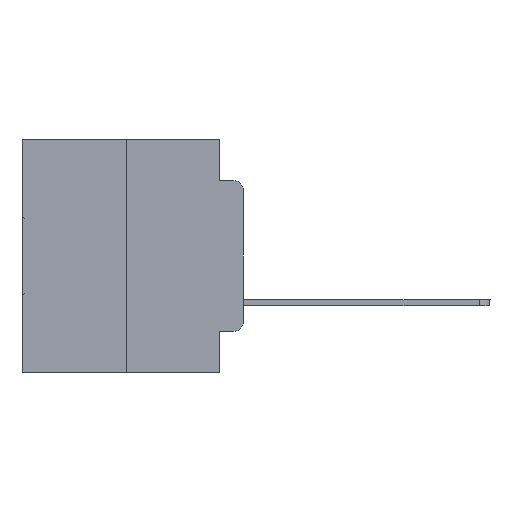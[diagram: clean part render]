
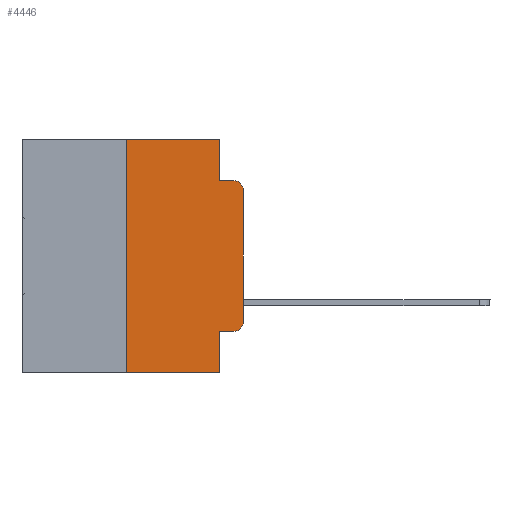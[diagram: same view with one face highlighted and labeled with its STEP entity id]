
A CAD part, left-side view. The second image highlights one B-rep face of the part: STEP entity #4446.
In plain terms, the highlighted planar face has unit normal (-1, 0, 0).
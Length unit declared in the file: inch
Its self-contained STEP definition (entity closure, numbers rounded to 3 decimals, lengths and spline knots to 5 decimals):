
#387 = VERTEX_POINT ( 'NONE', #19240 ) ;
#478 = EDGE_CURVE ( 'NONE', #12001, #10511, #5545, .T. ) ;
#784 = CARTESIAN_POINT ( 'NONE',  ( 0., 0.051, -0.4115 ) ) ;
#855 = VERTEX_POINT ( 'NONE', #19001 ) ;
#1096 = CARTESIAN_POINT ( 'NONE',  ( 0., 0.25, 0. ) ) ;
#1797 = LINE ( 'NONE', #3790, #17445 ) ;
#2346 = EDGE_CURVE ( 'NONE', #4085, #24721, #22886, .T. ) ;
#2978 = CARTESIAN_POINT ( 'NONE',  ( 0., 0.051, 0. ) ) ;
#3508 = CARTESIAN_POINT ( 'NONE',  ( 0., 0.051, 0. ) ) ;
#3790 = CARTESIAN_POINT ( 'NONE',  ( 0., 0.051, -0.0885 ) ) ;
#4085 = VERTEX_POINT ( 'NONE', #2978 ) ;
#4171 = ORIENTED_EDGE ( 'NONE', *, *, #13759, .T. ) ;
#4347 = VECTOR ( 'NONE', #24186, 39.37008 ) ;
#4446 = ADVANCED_FACE ( 'NONE', ( #16095 ), #20262, .F. ) ;
#5102 = DIRECTION ( 'NONE',  ( 0., 0., -1. ) ) ;
#5545 = LINE ( 'NONE', #1096, #15747 ) ;
#6130 = ORIENTED_EDGE ( 'NONE', *, *, #12969, .T. ) ;
#6351 = ORIENTED_EDGE ( 'NONE', *, *, #13719, .F. ) ;
#6355 = VECTOR ( 'NONE', #13452, 39.37008 ) ;
#6681 = CARTESIAN_POINT ( 'NONE',  ( 0., 0.25, -0.5 ) ) ;
#7059 = AXIS2_PLACEMENT_3D ( 'NONE', #24426, #24642, #22497 ) ;
#7614 = AXIS2_PLACEMENT_3D ( 'NONE', #11608, #21260, #5102 ) ;
#7624 = VECTOR ( 'NONE', #13855, 39.37008 ) ;
#8023 = VECTOR ( 'NONE', #24459, 39.37008 ) ;
#9468 = CARTESIAN_POINT ( 'NONE',  ( 0., 0.02, -0.1085 ) ) ;
#9555 = ORIENTED_EDGE ( 'NONE', *, *, #25316, .T. ) ;
#9809 = CARTESIAN_POINT ( 'NONE',  ( 0., 0.051, -0.4115 ) ) ;
#10511 = VERTEX_POINT ( 'NONE', #12247 ) ;
#10551 = LINE ( 'NONE', #784, #4347 ) ;
#11219 = CARTESIAN_POINT ( 'NONE',  ( 0., 0.473, -0.5 ) ) ;
#11608 = CARTESIAN_POINT ( 'NONE',  ( 0., 0.02, -0.3915 ) ) ;
#11614 = ORIENTED_EDGE ( 'NONE', *, *, #23508, .T. ) ;
#12001 = VERTEX_POINT ( 'NONE', #6681 ) ;
#12176 = DIRECTION ( 'NONE',  ( 0., 0., 1. ) ) ;
#12247 = CARTESIAN_POINT ( 'NONE',  ( 0., 0.25, 0. ) ) ;
#12268 = LINE ( 'NONE', #17048, #21388 ) ;
#12561 = VERTEX_POINT ( 'NONE', #15906 ) ;
#12969 = EDGE_CURVE ( 'NONE', #25031, #12561, #14559, .T. ) ;
#13251 = LINE ( 'NONE', #11219, #6355 ) ;
#13452 = DIRECTION ( 'NONE',  ( 0., -1., 0. ) ) ;
#13719 = EDGE_CURVE ( 'NONE', #24721, #12561, #1797, .T. ) ;
#13759 = EDGE_CURVE ( 'NONE', #27956, #27837, #10551, .T. ) ;
#13766 = VECTOR ( 'NONE', #25770, 39.37008 ) ;
#13855 = DIRECTION ( 'NONE',  ( 0., 0., -1. ) ) ;
#13918 = EDGE_LOOP ( 'NONE', ( #11614, #6130, #6351, #15587, #24100, #21765, #9555, #19678, #4171, #14757 ) ) ;
#14559 = CIRCLE ( 'NONE', #15472, 0.02 ) ;
#14757 = ORIENTED_EDGE ( 'NONE', *, *, #17914, .T. ) ;
#15472 = AXIS2_PLACEMENT_3D ( 'NONE', #9468, #25727, #21134 ) ;
#15587 = ORIENTED_EDGE ( 'NONE', *, *, #2346, .F. ) ;
#15747 = VECTOR ( 'NONE', #17697, 39.37008 ) ;
#15906 = CARTESIAN_POINT ( 'NONE',  ( 0., 0.02, -0.0885 ) ) ;
#16095 = FACE_OUTER_BOUND ( 'NONE', #13918, .T. ) ;
#16406 = CARTESIAN_POINT ( 'NONE',  ( 0., 0.02, -0.4115 ) ) ;
#16682 = LINE ( 'NONE', #25470, #13766 ) ;
#17048 = CARTESIAN_POINT ( 'NONE',  ( 0., 0., 0. ) ) ;
#17445 = VECTOR ( 'NONE', #19388, 39.37008 ) ;
#17697 = DIRECTION ( 'NONE',  ( 0., 0., 1. ) ) ;
#17914 = EDGE_CURVE ( 'NONE', #27837, #387, #19156, .T. ) ;
#18411 = CARTESIAN_POINT ( 'NONE',  ( 0., 0.051, -0.0885 ) ) ;
#19001 = CARTESIAN_POINT ( 'NONE',  ( 0., 0.051, -0.5 ) ) ;
#19156 = CIRCLE ( 'NONE', #7614, 0.02 ) ;
#19240 = CARTESIAN_POINT ( 'NONE',  ( 0., 0., -0.3915 ) ) ;
#19388 = DIRECTION ( 'NONE',  ( 0., -1., 0. ) ) ;
#19678 = ORIENTED_EDGE ( 'NONE', *, *, #29385, .F. ) ;
#20262 = PLANE ( 'NONE',  #7059 ) ;
#21134 = DIRECTION ( 'NONE',  ( 0., 0., -1. ) ) ;
#21260 = DIRECTION ( 'NONE',  ( -1., 0., 0. ) ) ;
#21388 = VECTOR ( 'NONE', #12176, 39.37008 ) ;
#21765 = ORIENTED_EDGE ( 'NONE', *, *, #478, .F. ) ;
#22497 = DIRECTION ( 'NONE',  ( 0., 0., -1. ) ) ;
#22704 = EDGE_CURVE ( 'NONE', #10511, #4085, #16682, .T. ) ;
#22886 = LINE ( 'NONE', #29630, #7624 ) ;
#23508 = EDGE_CURVE ( 'NONE', #387, #25031, #12268, .T. ) ;
#24100 = ORIENTED_EDGE ( 'NONE', *, *, #22704, .F. ) ;
#24186 = DIRECTION ( 'NONE',  ( 0., -1., 0. ) ) ;
#24426 = CARTESIAN_POINT ( 'NONE',  ( 0., 0.473, 0. ) ) ;
#24459 = DIRECTION ( 'NONE',  ( 0., 0., -1. ) ) ;
#24642 = DIRECTION ( 'NONE',  ( 1., 0., 0. ) ) ;
#24721 = VERTEX_POINT ( 'NONE', #18411 ) ;
#25031 = VERTEX_POINT ( 'NONE', #26668 ) ;
#25316 = EDGE_CURVE ( 'NONE', #12001, #855, #13251, .T. ) ;
#25470 = CARTESIAN_POINT ( 'NONE',  ( 0., 0.473, 0. ) ) ;
#25727 = DIRECTION ( 'NONE',  ( -1., 0., 0. ) ) ;
#25770 = DIRECTION ( 'NONE',  ( 0., -1., 0. ) ) ;
#26668 = CARTESIAN_POINT ( 'NONE',  ( 0., 0., -0.1085 ) ) ;
#27837 = VERTEX_POINT ( 'NONE', #16406 ) ;
#27956 = VERTEX_POINT ( 'NONE', #9809 ) ;
#29385 = EDGE_CURVE ( 'NONE', #27956, #855, #29820, .T. ) ;
#29630 = CARTESIAN_POINT ( 'NONE',  ( 0., 0.051, 0. ) ) ;
#29820 = LINE ( 'NONE', #3508, #8023 ) ;
